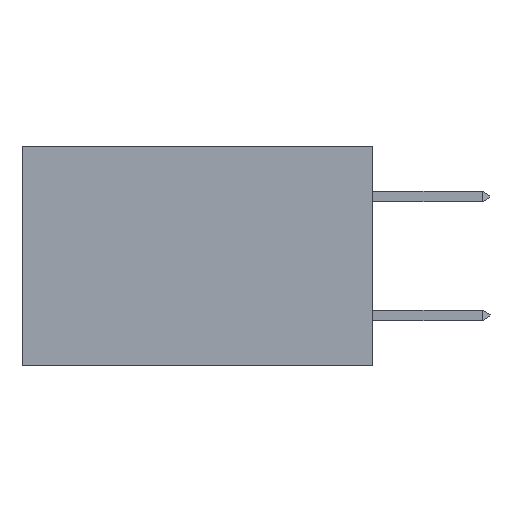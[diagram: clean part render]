
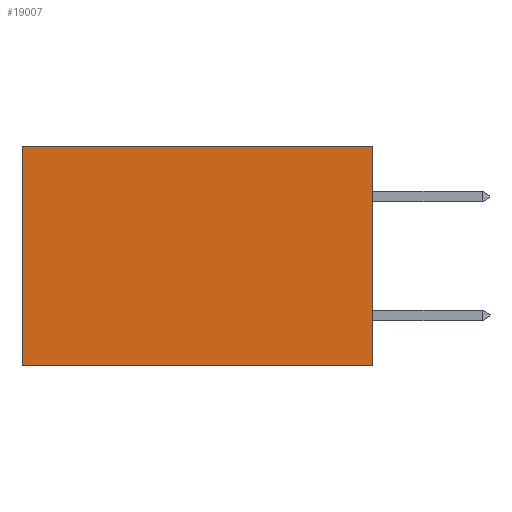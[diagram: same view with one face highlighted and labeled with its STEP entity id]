
A CAD part, left-side view. The second image highlights one B-rep face of the part: STEP entity #19007.
In plain terms, the highlighted planar face has unit normal (-1, 0, 0).
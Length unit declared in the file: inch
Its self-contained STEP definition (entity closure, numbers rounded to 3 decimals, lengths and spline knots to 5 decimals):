
#156 = DIRECTION ( 'NONE',  ( 0., 0., -1. ) ) ;
#1019 = CARTESIAN_POINT ( 'NONE',  ( 0.277, 0., -0.37 ) ) ;
#2007 = DIRECTION ( 'NONE',  ( 0., 1., 0. ) ) ;
#2441 = EDGE_CURVE ( 'NONE', #4574, #10414, #34807, .T. ) ;
#2860 = LINE ( 'NONE', #32550, #30821 ) ;
#2911 = VECTOR ( 'NONE', #6903, 39.37008 ) ;
#3676 = DIRECTION ( 'NONE',  ( 1., 0., 0. ) ) ;
#3682 = VECTOR ( 'NONE', #27175, 39.37008 ) ;
#4153 = CARTESIAN_POINT ( 'NONE',  ( 0.277, 0., 0. ) ) ;
#4574 = VERTEX_POINT ( 'NONE', #33164 ) ;
#6903 = DIRECTION ( 'NONE',  ( 0., 1., 0. ) ) ;
#8172 = CARTESIAN_POINT ( 'NONE',  ( 0.277, 0.59, -0.37 ) ) ;
#8875 = VERTEX_POINT ( 'NONE', #12904 ) ;
#9046 = EDGE_CURVE ( 'NONE', #22487, #10414, #31666, .T. ) ;
#9065 = EDGE_CURVE ( 'NONE', #8875, #4574, #2860, .T. ) ;
#10414 = VERTEX_POINT ( 'NONE', #16059 ) ;
#12904 = CARTESIAN_POINT ( 'NONE',  ( 0.277, 0., 0. ) ) ;
#14069 = VECTOR ( 'NONE', #2007, 39.37008 ) ;
#14497 = ORIENTED_EDGE ( 'NONE', *, *, #20846, .T. ) ;
#16059 = CARTESIAN_POINT ( 'NONE',  ( 0.277, 0.59, -0.37 ) ) ;
#17342 = LINE ( 'NONE', #4153, #2911 ) ;
#17854 = ORIENTED_EDGE ( 'NONE', *, *, #9065, .F. ) ;
#18875 = EDGE_LOOP ( 'NONE', ( #25266, #24432, #17854, #14497 ) ) ;
#19007 = ADVANCED_FACE ( 'NONE', ( #19985 ), #19899, .F. ) ;
#19899 = PLANE ( 'NONE',  #22249 ) ;
#19985 = FACE_OUTER_BOUND ( 'NONE', #18875, .T. ) ;
#20846 = EDGE_CURVE ( 'NONE', #8875, #22487, #17342, .T. ) ;
#22249 = AXIS2_PLACEMENT_3D ( 'NONE', #1019, #3676, #22673 ) ;
#22439 = CARTESIAN_POINT ( 'NONE',  ( 0.277, 0., -0.37 ) ) ;
#22487 = VERTEX_POINT ( 'NONE', #24232 ) ;
#22673 = DIRECTION ( 'NONE',  ( 0., 0., -1. ) ) ;
#24232 = CARTESIAN_POINT ( 'NONE',  ( 0.277, 0.59, 0. ) ) ;
#24432 = ORIENTED_EDGE ( 'NONE', *, *, #2441, .F. ) ;
#25266 = ORIENTED_EDGE ( 'NONE', *, *, #9046, .T. ) ;
#27175 = DIRECTION ( 'NONE',  ( 0., 0., -1. ) ) ;
#30821 = VECTOR ( 'NONE', #156, 39.37008 ) ;
#31666 = LINE ( 'NONE', #8172, #3682 ) ;
#32550 = CARTESIAN_POINT ( 'NONE',  ( 0.277, 0., -0.37 ) ) ;
#33164 = CARTESIAN_POINT ( 'NONE',  ( 0.277, 0., -0.37 ) ) ;
#34807 = LINE ( 'NONE', #22439, #14069 ) ;
